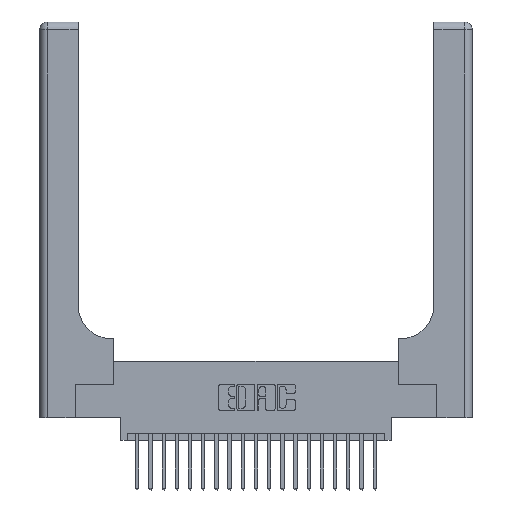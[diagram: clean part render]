
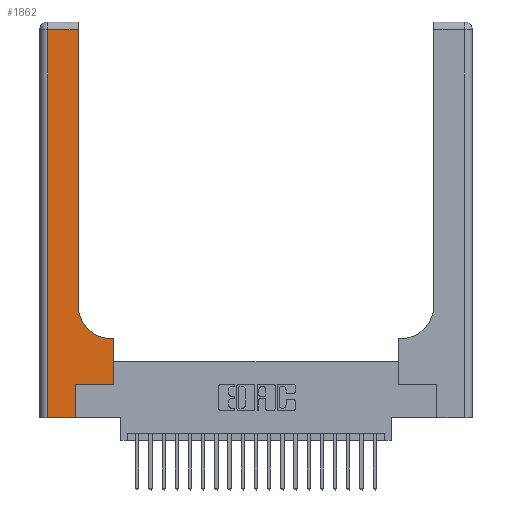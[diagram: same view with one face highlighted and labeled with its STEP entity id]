
A CAD part, top view. The second image highlights one B-rep face of the part: STEP entity #1862.
In plain terms, the highlighted planar face has unit normal (0, 0, 1).
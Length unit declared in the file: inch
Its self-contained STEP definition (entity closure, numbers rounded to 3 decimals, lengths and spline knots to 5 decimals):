
#454 = ORIENTED_EDGE ( 'NONE', *, *, #3232, .T. ) ;
#635 = VERTEX_POINT ( 'NONE', #8973 ) ;
#749 = LINE ( 'NONE', #1717, #19452 ) ;
#759 = EDGE_CURVE ( 'NONE', #6453, #14948, #15414, .T. ) ;
#930 = ORIENTED_EDGE ( 'NONE', *, *, #12959, .T. ) ;
#983 = LINE ( 'NONE', #1988, #10188 ) ;
#1717 = CARTESIAN_POINT ( 'NONE',  ( 0.5585, 0.25, 0.37 ) ) ;
#1862 = ADVANCED_FACE ( 'NONE', ( #18399 ), #13458, .F. ) ;
#1975 = CARTESIAN_POINT ( 'NONE',  ( 0., 0., 0.37 ) ) ;
#1988 = CARTESIAN_POINT ( 'NONE',  ( 0.269, 0., 0.37 ) ) ;
#2295 = AXIS2_PLACEMENT_3D ( 'NONE', #17667, #17455, #17305 ) ;
#2443 = LINE ( 'NONE', #4436, #16883 ) ;
#2595 = CARTESIAN_POINT ( 'NONE',  ( 0.5585, 0.25, 0.37 ) ) ;
#2964 = EDGE_LOOP ( 'NONE', ( #11309, #10466, #15078, #14400, #16953, #930, #454, #6246, #18149 ) ) ;
#3232 = EDGE_CURVE ( 'NONE', #20436, #21695, #749, .T. ) ;
#3333 = CARTESIAN_POINT ( 'NONE',  ( 0.06, 2.94, 0.37 ) ) ;
#3399 = AXIS2_PLACEMENT_3D ( 'NONE', #13368, #13306, #13282 ) ;
#3835 = DIRECTION ( 'NONE',  ( 0., 1., 0. ) ) ;
#4436 = CARTESIAN_POINT ( 'NONE',  ( 0., 2.94, 0.37 ) ) ;
#4622 = VECTOR ( 'NONE', #7856, 39.37008 ) ;
#4653 = EDGE_CURVE ( 'NONE', #15774, #22933, #10797, .T. ) ;
#4675 = CARTESIAN_POINT ( 'NONE',  ( 0.269, 0.25, 0.37 ) ) ;
#5101 = VERTEX_POINT ( 'NONE', #3333 ) ;
#5102 = DIRECTION ( 'NONE',  ( 0., 1., 0. ) ) ;
#5361 = EDGE_CURVE ( 'NONE', #635, #5101, #2443, .T. ) ;
#5405 = DIRECTION ( 'NONE',  ( 0., 1., 0. ) ) ;
#5692 = LINE ( 'NONE', #4675, #14799 ) ;
#6190 = DIRECTION ( 'NONE',  ( -1., 0., 0. ) ) ;
#6246 = ORIENTED_EDGE ( 'NONE', *, *, #6975, .T. ) ;
#6453 = VERTEX_POINT ( 'NONE', #8366 ) ;
#6975 = EDGE_CURVE ( 'NONE', #21695, #6453, #10069, .T. ) ;
#7476 = DIRECTION ( 'NONE',  ( 0., -1., 0. ) ) ;
#7856 = DIRECTION ( 'NONE',  ( -1., 0., 0. ) ) ;
#8036 = EDGE_CURVE ( 'NONE', #5101, #15774, #14270, .T. ) ;
#8366 = CARTESIAN_POINT ( 'NONE',  ( 0.5415, 0.6, 0.37 ) ) ;
#8510 = CARTESIAN_POINT ( 'NONE',  ( 0.269, 0., 0.37 ) ) ;
#8973 = CARTESIAN_POINT ( 'NONE',  ( 0.2915, 2.94, 0.37 ) ) ;
#9363 = DIRECTION ( 'NONE',  ( 1., 0., 0. ) ) ;
#10069 = LINE ( 'NONE', #18566, #4622 ) ;
#10188 = VECTOR ( 'NONE', #3835, 39.37008 ) ;
#10441 = VERTEX_POINT ( 'NONE', #21280 ) ;
#10466 = ORIENTED_EDGE ( 'NONE', *, *, #5361, .T. ) ;
#10797 = LINE ( 'NONE', #1975, #15015 ) ;
#11309 = ORIENTED_EDGE ( 'NONE', *, *, #21803, .T. ) ;
#12043 = CARTESIAN_POINT ( 'NONE',  ( 0.5585, 0.6, 0.37 ) ) ;
#12959 = EDGE_CURVE ( 'NONE', #10441, #20436, #5692, .T. ) ;
#13147 = VECTOR ( 'NONE', #7476, 39.37008 ) ;
#13282 = DIRECTION ( 'NONE',  ( -1., 0., 0. ) ) ;
#13306 = DIRECTION ( 'NONE',  ( 0., 0., -1. ) ) ;
#13368 = CARTESIAN_POINT ( 'NONE',  ( 0., 3., 0.37 ) ) ;
#13458 = PLANE ( 'NONE',  #3399 ) ;
#14270 = LINE ( 'NONE', #16505, #13147 ) ;
#14400 = ORIENTED_EDGE ( 'NONE', *, *, #4653, .T. ) ;
#14799 = VECTOR ( 'NONE', #15540, 39.37008 ) ;
#14948 = VERTEX_POINT ( 'NONE', #17266 ) ;
#15015 = VECTOR ( 'NONE', #9363, 39.37008 ) ;
#15078 = ORIENTED_EDGE ( 'NONE', *, *, #8036, .T. ) ;
#15414 = CIRCLE ( 'NONE', #2295, 0.25 ) ;
#15540 = DIRECTION ( 'NONE',  ( 1., 0., 0. ) ) ;
#15774 = VERTEX_POINT ( 'NONE', #21950 ) ;
#16505 = CARTESIAN_POINT ( 'NONE',  ( 0.06, 3., 0.37 ) ) ;
#16883 = VECTOR ( 'NONE', #6190, 39.37008 ) ;
#16953 = ORIENTED_EDGE ( 'NONE', *, *, #21316, .T. ) ;
#17266 = CARTESIAN_POINT ( 'NONE',  ( 0.2915, 0.85, 0.37 ) ) ;
#17305 = DIRECTION ( 'NONE',  ( 1., 0., 0. ) ) ;
#17455 = DIRECTION ( 'NONE',  ( 0., 0., -1. ) ) ;
#17667 = CARTESIAN_POINT ( 'NONE',  ( 0.5415, 0.85, 0.37 ) ) ;
#17699 = CARTESIAN_POINT ( 'NONE',  ( 0.2915, 3., 0.37 ) ) ;
#18149 = ORIENTED_EDGE ( 'NONE', *, *, #759, .T. ) ;
#18399 = FACE_OUTER_BOUND ( 'NONE', #2964, .T. ) ;
#18566 = CARTESIAN_POINT ( 'NONE',  ( 0.2915, 0.6, 0.37 ) ) ;
#19086 = VECTOR ( 'NONE', #5102, 39.37008 ) ;
#19452 = VECTOR ( 'NONE', #5405, 39.37008 ) ;
#19647 = LINE ( 'NONE', #17699, #19086 ) ;
#20436 = VERTEX_POINT ( 'NONE', #2595 ) ;
#21280 = CARTESIAN_POINT ( 'NONE',  ( 0.269, 0.25, 0.37 ) ) ;
#21316 = EDGE_CURVE ( 'NONE', #22933, #10441, #983, .T. ) ;
#21695 = VERTEX_POINT ( 'NONE', #12043 ) ;
#21803 = EDGE_CURVE ( 'NONE', #14948, #635, #19647, .T. ) ;
#21950 = CARTESIAN_POINT ( 'NONE',  ( 0.06, 0., 0.37 ) ) ;
#22933 = VERTEX_POINT ( 'NONE', #8510 ) ;
